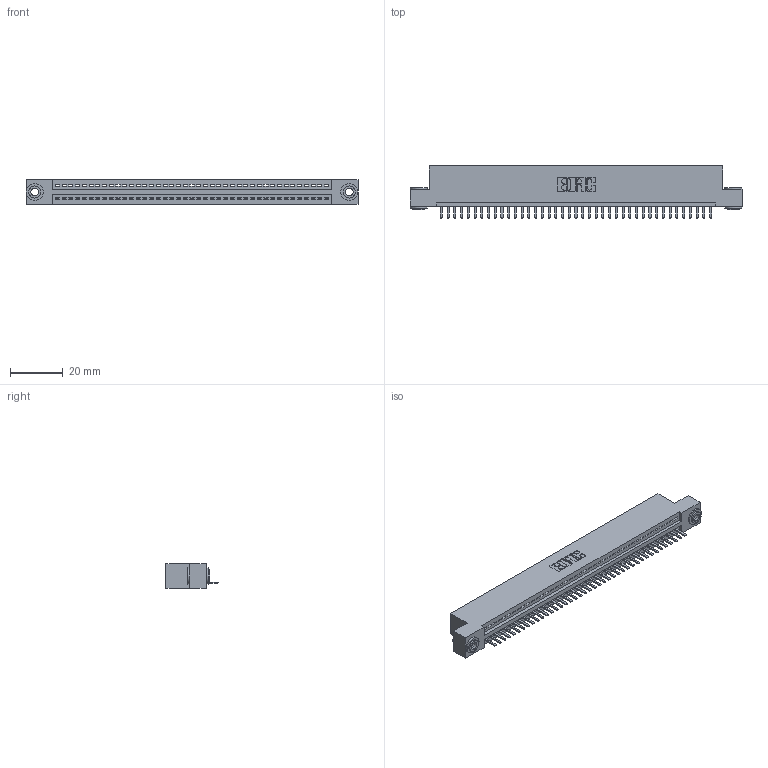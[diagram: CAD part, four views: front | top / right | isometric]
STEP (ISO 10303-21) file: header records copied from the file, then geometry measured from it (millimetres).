
FILE_DESCRIPTION (( 'STEP AP203' ), '1' );
FILE_NAME ('345-041-520-103.STEP', '2018-09-05T06:56:02', ( '' ), ( '' ), 'SwSTEP 2.0', 'SolidWorks 2016', '' );
FILE_SCHEMA (( 'CONFIG_CONTROL_DESIGN' ));
Length unit declared in the file: inch
Products named in the file (4): 345 Part_Flush Mounting Lugs - 0.156 Dia-TH; 345-292-001_345-293-120; 345-250-002_345-250-002-102; 345-041-520-103
Assembly tree (44 placements, depth 2):
  345-041-520-103
    345 Part_Flush Mounting Lugs - 0.156 Dia-TH
    345-292-001_345-293-120  x41
    345-250-002_345-250-002-102  x2
Bounding box: 125.35 x 19.68 x 9.4 mm (x, y, z)
Volume: 11799 mm3; surface area: 15494.9 mm2
Topology: 44 solids, 44 shells, 2706 faces, 7961 edges, 5194 vertices
Faces by surface type: plane 1812, cylinder 886, cone 8
Entity records: 31756 total; most frequent: CARTESIAN_POINT 5490, ORIENTED_EDGE 5446, DIRECTION 4815, EDGE_CURVE 2723, VECTOR 2399, LINE 2399, VERTEX_POINT 1810, AXIS2_PLACEMENT_3D 1208
